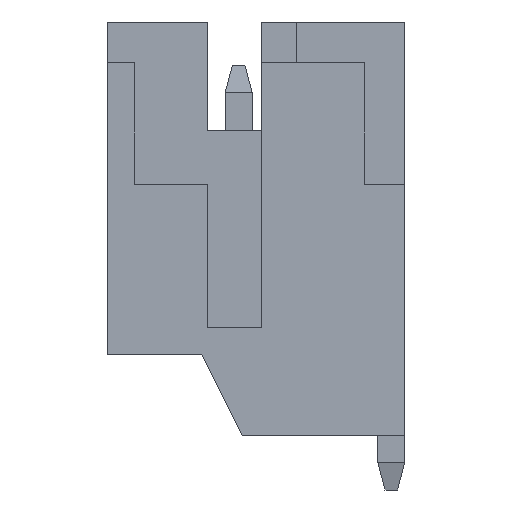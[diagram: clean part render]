
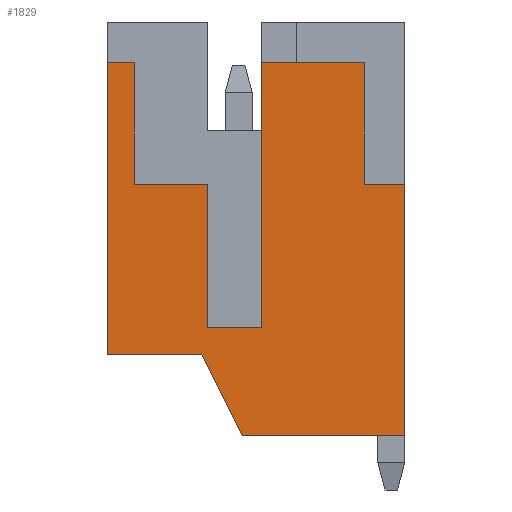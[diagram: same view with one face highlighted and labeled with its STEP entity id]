
A CAD part, left-side view. The second image highlights one B-rep face of the part: STEP entity #1829.
In plain terms, the highlighted planar face has unit normal (-1, 0, 0).
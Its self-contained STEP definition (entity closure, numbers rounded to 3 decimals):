
#648 = EDGE_CURVE ( 'NONE', #10554, #11697, #7031, .T. ) ;
#997 = VERTEX_POINT ( 'NONE', #9121 ) ;
#1085 = VERTEX_POINT ( 'NONE', #8342 ) ;
#1216 = VECTOR ( 'NONE', #6637, 1000. ) ;
#1398 = DIRECTION ( 'NONE',  ( 0., 0., -1. ) ) ;
#1523 = DIRECTION ( 'NONE',  ( 0., -1., 0. ) ) ;
#1679 = DIRECTION ( 'NONE',  ( -1., 0., 0. ) ) ;
#1774 = CARTESIAN_POINT ( 'NONE',  ( -3., -0.42, 0.5 ) ) ;
#1829 = ADVANCED_FACE ( 'NONE', ( #10499 ), #10964, .T. ) ;
#1871 = CARTESIAN_POINT ( 'NONE',  ( -3., -2.32, 3.15 ) ) ;
#1903 = EDGE_CURVE ( 'NONE', #10554, #4389, #5818, .T. ) ;
#1917 = DIRECTION ( 'NONE',  ( 0., 0., -1. ) ) ;
#1924 = DIRECTION ( 'NONE',  ( 0., -0.447, -0.894 ) ) ;
#2188 = VECTOR ( 'NONE', #6351, 1000. ) ;
#2345 = EDGE_CURVE ( 'NONE', #2469, #7050, #3314, .T. ) ;
#2469 = VERTEX_POINT ( 'NONE', #2828 ) ;
#2509 = EDGE_CURVE ( 'NONE', #8953, #5091, #3471, .T. ) ;
#2575 = LINE ( 'NONE', #9802, #3445 ) ;
#2621 = LINE ( 'NONE', #3864, #11084 ) ;
#2793 = ORIENTED_EDGE ( 'NONE', *, *, #1903, .F. ) ;
#2828 = CARTESIAN_POINT ( 'NONE',  ( -3., 0.58, 0.5 ) ) ;
#2839 = ORIENTED_EDGE ( 'NONE', *, *, #648, .T. ) ;
#2885 = VERTEX_POINT ( 'NONE', #6963 ) ;
#2922 = EDGE_CURVE ( 'NONE', #2885, #4771, #10906, .T. ) ;
#2927 = ORIENTED_EDGE ( 'NONE', *, *, #11386, .T. ) ;
#3137 = EDGE_CURVE ( 'NONE', #11697, #997, #6814, .T. ) ;
#3144 = VECTOR ( 'NONE', #1917, 1000. ) ;
#3177 = LINE ( 'NONE', #9021, #11061 ) ;
#3314 = LINE ( 'NONE', #7137, #7838 ) ;
#3368 = DIRECTION ( 'NONE',  ( 0., 1., 0. ) ) ;
#3396 = VERTEX_POINT ( 'NONE', #10667 ) ;
#3445 = VECTOR ( 'NONE', #11719, 1000. ) ;
#3448 = CARTESIAN_POINT ( 'NONE',  ( -3., -0.07, -1.5 ) ) ;
#3471 = LINE ( 'NONE', #4571, #10773 ) ;
#3543 = DIRECTION ( 'NONE',  ( 0., -1., 0. ) ) ;
#3637 = ORIENTED_EDGE ( 'NONE', *, *, #6093, .T. ) ;
#3710 = DIRECTION ( 'NONE',  ( 0., 1., 0. ) ) ;
#3781 = DIRECTION ( 'NONE',  ( 0., -1., 0. ) ) ;
#3790 = CARTESIAN_POINT ( 'NONE',  ( -3., 1.93, 3.15 ) ) ;
#3864 = CARTESIAN_POINT ( 'NONE',  ( -3., 2.43, 0. ) ) ;
#3920 = VECTOR ( 'NONE', #3710, 1000. ) ;
#4194 = CARTESIAN_POINT ( 'NONE',  ( -3., -3.07, 5.4 ) ) ;
#4389 = VERTEX_POINT ( 'NONE', #12020 ) ;
#4571 = CARTESIAN_POINT ( 'NONE',  ( -3., -0.07, -1.5 ) ) ;
#4771 = VERTEX_POINT ( 'NONE', #6681 ) ;
#4800 = CARTESIAN_POINT ( 'NONE',  ( -3., 2.43, 6.15 ) ) ;
#5053 = VECTOR ( 'NONE', #3368, 1000. ) ;
#5091 = VERTEX_POINT ( 'NONE', #3448 ) ;
#5152 = VERTEX_POINT ( 'NONE', #5508 ) ;
#5171 = LINE ( 'NONE', #4800, #3144 ) ;
#5209 = ORIENTED_EDGE ( 'NONE', *, *, #10874, .T. ) ;
#5331 = LINE ( 'NONE', #11682, #11751 ) ;
#5368 = EDGE_CURVE ( 'NONE', #1085, #8953, #2621, .T. ) ;
#5508 = CARTESIAN_POINT ( 'NONE',  ( -3., -2.32, 3.15 ) ) ;
#5514 = CARTESIAN_POINT ( 'NONE',  ( -3., 1.93, 5.4 ) ) ;
#5640 = DIRECTION ( 'NONE',  ( 0., -1., 0. ) ) ;
#5818 = LINE ( 'NONE', #6423, #2188 ) ;
#5845 = ORIENTED_EDGE ( 'NONE', *, *, #6796, .F. ) ;
#6093 = EDGE_CURVE ( 'NONE', #3396, #10625, #7694, .T. ) ;
#6274 = DIRECTION ( 'NONE',  ( 0., -1., 0. ) ) ;
#6351 = DIRECTION ( 'NONE',  ( 0., -1., 0. ) ) ;
#6423 = CARTESIAN_POINT ( 'NONE',  ( -3., -0.42, 3.15 ) ) ;
#6425 = CARTESIAN_POINT ( 'NONE',  ( -3., -3.07, 5.4 ) ) ;
#6637 = DIRECTION ( 'NONE',  ( 0., 0., 1. ) ) ;
#6646 = VECTOR ( 'NONE', #1523, 1000. ) ;
#6681 = CARTESIAN_POINT ( 'NONE',  ( -3., -0.42, 5.4 ) ) ;
#6761 = ORIENTED_EDGE ( 'NONE', *, *, #7972, .T. ) ;
#6796 = EDGE_CURVE ( 'NONE', #4389, #2469, #2575, .T. ) ;
#6814 = LINE ( 'NONE', #6425, #3920 ) ;
#6963 = CARTESIAN_POINT ( 'NONE',  ( -3., -2.32, 5.4 ) ) ;
#7031 = LINE ( 'NONE', #3790, #1216 ) ;
#7050 = VERTEX_POINT ( 'NONE', #1774 ) ;
#7137 = CARTESIAN_POINT ( 'NONE',  ( -3., -0.42, 0.5 ) ) ;
#7202 = CARTESIAN_POINT ( 'NONE',  ( -3., -3.07, 6.15 ) ) ;
#7239 = CARTESIAN_POINT ( 'NONE',  ( -3., 0., 0. ) ) ;
#7287 = DIRECTION ( 'NONE',  ( 0., 0., 1. ) ) ;
#7337 = ORIENTED_EDGE ( 'NONE', *, *, #3137, .T. ) ;
#7694 = LINE ( 'NONE', #7202, #8428 ) ;
#7785 = EDGE_CURVE ( 'NONE', #5091, #3396, #9125, .T. ) ;
#7838 = VECTOR ( 'NONE', #6274, 1000. ) ;
#7972 = EDGE_CURVE ( 'NONE', #997, #1085, #5171, .T. ) ;
#8001 = CARTESIAN_POINT ( 'NONE',  ( -3., 0.68, 0. ) ) ;
#8064 = CARTESIAN_POINT ( 'NONE',  ( -3., -3.07, -1.5 ) ) ;
#8342 = CARTESIAN_POINT ( 'NONE',  ( -3., 2.43, 0. ) ) ;
#8428 = VECTOR ( 'NONE', #10768, 1000. ) ;
#8650 = LINE ( 'NONE', #1871, #10829 ) ;
#8670 = CARTESIAN_POINT ( 'NONE',  ( -3., 1.93, 3.15 ) ) ;
#8953 = VERTEX_POINT ( 'NONE', #8001 ) ;
#9021 = CARTESIAN_POINT ( 'NONE',  ( -3., -2.32, 3.15 ) ) ;
#9121 = CARTESIAN_POINT ( 'NONE',  ( -3., 2.43, 5.4 ) ) ;
#9125 = LINE ( 'NONE', #8064, #6646 ) ;
#9346 = AXIS2_PLACEMENT_3D ( 'NONE', #7239, #1679, #3543 ) ;
#9532 = ORIENTED_EDGE ( 'NONE', *, *, #9829, .F. ) ;
#9802 = CARTESIAN_POINT ( 'NONE',  ( -3., 0.58, 3.15 ) ) ;
#9829 = EDGE_CURVE ( 'NONE', #5152, #10625, #8650, .T. ) ;
#10026 = ORIENTED_EDGE ( 'NONE', *, *, #5368, .T. ) ;
#10283 = EDGE_LOOP ( 'NONE', ( #7337, #6761, #10026, #10686, #11321, #3637, #9532, #5209, #10552, #2927, #11742, #5845, #2793, #2839 ) ) ;
#10499 = FACE_OUTER_BOUND ( 'NONE', #10283, .T. ) ;
#10552 = ORIENTED_EDGE ( 'NONE', *, *, #2922, .T. ) ;
#10554 = VERTEX_POINT ( 'NONE', #8670 ) ;
#10574 = CARTESIAN_POINT ( 'NONE',  ( -3., -3.07, 3.15 ) ) ;
#10625 = VERTEX_POINT ( 'NONE', #10574 ) ;
#10667 = CARTESIAN_POINT ( 'NONE',  ( -3., -3.07, -1.5 ) ) ;
#10686 = ORIENTED_EDGE ( 'NONE', *, *, #2509, .T. ) ;
#10768 = DIRECTION ( 'NONE',  ( 0., 0., 1. ) ) ;
#10773 = VECTOR ( 'NONE', #1924, 1000. ) ;
#10829 = VECTOR ( 'NONE', #3781, 1000. ) ;
#10874 = EDGE_CURVE ( 'NONE', #5152, #2885, #3177, .T. ) ;
#10906 = LINE ( 'NONE', #4194, #5053 ) ;
#10964 = PLANE ( 'NONE',  #9346 ) ;
#11061 = VECTOR ( 'NONE', #7287, 1000. ) ;
#11084 = VECTOR ( 'NONE', #5640, 1000. ) ;
#11321 = ORIENTED_EDGE ( 'NONE', *, *, #7785, .T. ) ;
#11386 = EDGE_CURVE ( 'NONE', #4771, #7050, #5331, .T. ) ;
#11682 = CARTESIAN_POINT ( 'NONE',  ( -3., -0.42, 6.15 ) ) ;
#11697 = VERTEX_POINT ( 'NONE', #5514 ) ;
#11719 = DIRECTION ( 'NONE',  ( 0., 0., -1. ) ) ;
#11742 = ORIENTED_EDGE ( 'NONE', *, *, #2345, .F. ) ;
#11751 = VECTOR ( 'NONE', #1398, 1000. ) ;
#12020 = CARTESIAN_POINT ( 'NONE',  ( -3., 0.58, 3.15 ) ) ;
